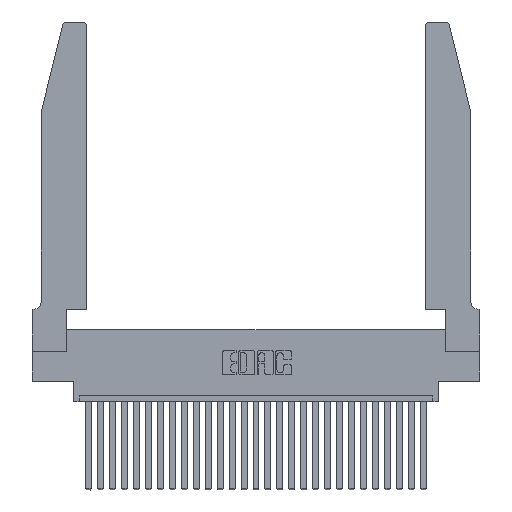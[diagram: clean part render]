
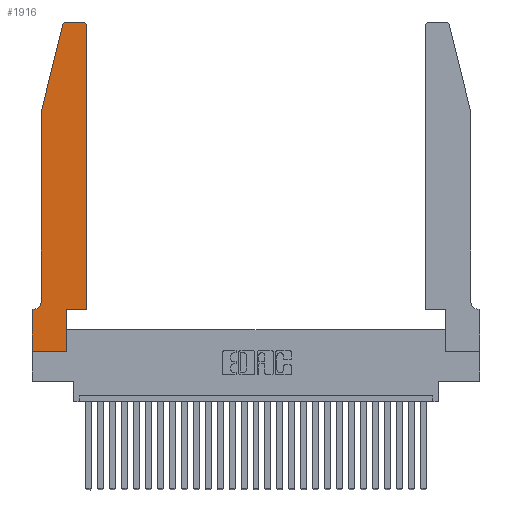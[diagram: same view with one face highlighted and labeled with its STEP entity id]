
A CAD part, top view. The second image highlights one B-rep face of the part: STEP entity #1916.
In plain terms, the highlighted planar face has unit normal (0, 0, 1).
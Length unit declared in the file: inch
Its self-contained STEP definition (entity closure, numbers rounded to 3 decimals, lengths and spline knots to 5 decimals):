
#500 = VERTEX_POINT ( 'NONE', #1086 ) ;
#628 = ORIENTED_EDGE ( 'NONE', *, *, #988, .T. ) ;
#988 = EDGE_CURVE ( 'NONE', #17002, #27458, #21247, .T. ) ;
#1086 = CARTESIAN_POINT ( 'NONE',  ( 0.0055, 0.35, 0.37 ) ) ;
#1126 = LINE ( 'NONE', #27932, #23735 ) ;
#1313 = DIRECTION ( 'NONE',  ( 0., 1., 0. ) ) ;
#1916 = ADVANCED_FACE ( 'NONE', ( #3417 ), #9056, .T. ) ;
#1995 = CARTESIAN_POINT ( 'NONE',  ( 0.4505, 0.35, 0.37 ) ) ;
#2101 = ORIENTED_EDGE ( 'NONE', *, *, #27405, .T. ) ;
#2316 = VECTOR ( 'NONE', #14322, 39.37008 ) ;
#2616 = CARTESIAN_POINT ( 'NONE',  ( 0.2605, 2.75, 0.37 ) ) ;
#2664 = DIRECTION ( 'NONE',  ( 0., -1., 0. ) ) ;
#3417 = FACE_OUTER_BOUND ( 'NONE', #25079, .T. ) ;
#3504 = EDGE_CURVE ( 'NONE', #11143, #8281, #8775, .T. ) ;
#3629 = DIRECTION ( 'NONE',  ( 0., 1., 0. ) ) ;
#4807 = EDGE_CURVE ( 'NONE', #21581, #500, #25152, .T. ) ;
#4892 = LINE ( 'NONE', #25205, #21672 ) ;
#4987 = DIRECTION ( 'NONE',  ( -1., 0., 0. ) ) ;
#4996 = CARTESIAN_POINT ( 'NONE',  ( 0.0755, 2., 0.37 ) ) ;
#5519 = AXIS2_PLACEMENT_3D ( 'NONE', #13324, #24188, #26760 ) ;
#5520 = VERTEX_POINT ( 'NONE', #14639 ) ;
#5659 = LINE ( 'NONE', #10145, #27556 ) ;
#5723 = ORIENTED_EDGE ( 'NONE', *, *, #15871, .T. ) ;
#5845 = CIRCLE ( 'NONE', #5519, 0.03 ) ;
#6104 = CARTESIAN_POINT ( 'NONE',  ( 0.4505, 0.35, 0.37 ) ) ;
#6282 = LINE ( 'NONE', #14754, #7245 ) ;
#7245 = VECTOR ( 'NONE', #10486, 39.37008 ) ;
#7622 = CARTESIAN_POINT ( 'NONE',  ( 0.2865, 0.35, 0.37 ) ) ;
#7676 = ORIENTED_EDGE ( 'NONE', *, *, #24217, .T. ) ;
#7936 = DIRECTION ( 'NONE',  ( -1., 0., 0. ) ) ;
#8152 = EDGE_CURVE ( 'NONE', #5520, #20333, #20514, .T. ) ;
#8167 = VERTEX_POINT ( 'NONE', #1995 ) ;
#8184 = DIRECTION ( 'NONE',  ( 1., 0., 0. ) ) ;
#8281 = VERTEX_POINT ( 'NONE', #17832 ) ;
#8543 = DIRECTION ( 'NONE',  ( 0., 0., 1. ) ) ;
#8602 = CARTESIAN_POINT ( 'NONE',  ( 0.0755, 0.42, 0.37 ) ) ;
#8775 = LINE ( 'NONE', #27477, #2316 ) ;
#9056 = PLANE ( 'NONE',  #27855 ) ;
#10145 = CARTESIAN_POINT ( 'NONE',  ( 0., 0., 0.37 ) ) ;
#10486 = DIRECTION ( 'NONE',  ( -0.239, -0.971, 0. ) ) ;
#10800 = CARTESIAN_POINT ( 'NONE',  ( 0., 0.35, 0.37 ) ) ;
#11143 = VERTEX_POINT ( 'NONE', #21629 ) ;
#11714 = LINE ( 'NONE', #6104, #22681 ) ;
#12067 = ORIENTED_EDGE ( 'NONE', *, *, #3504, .T. ) ;
#12732 = DIRECTION ( 'NONE',  ( 1., 0., 0. ) ) ;
#13299 = VECTOR ( 'NONE', #4987, 39.37008 ) ;
#13324 = CARTESIAN_POINT ( 'NONE',  ( 0.284, 2.72, 0.37 ) ) ;
#13483 = ORIENTED_EDGE ( 'NONE', *, *, #20026, .T. ) ;
#13984 = ORIENTED_EDGE ( 'NONE', *, *, #26946, .T. ) ;
#14322 = DIRECTION ( 'NONE',  ( 0., -1., 0. ) ) ;
#14639 = CARTESIAN_POINT ( 'NONE',  ( 0.2865, 0., 0.37 ) ) ;
#14754 = CARTESIAN_POINT ( 'NONE',  ( 0.0755, 2., 0.37 ) ) ;
#15560 = VERTEX_POINT ( 'NONE', #4996 ) ;
#15871 = EDGE_CURVE ( 'NONE', #27236, #17002, #22140, .T. ) ;
#16231 = ORIENTED_EDGE ( 'NONE', *, *, #4807, .T. ) ;
#17002 = VERTEX_POINT ( 'NONE', #25467 ) ;
#17112 = AXIS2_PLACEMENT_3D ( 'NONE', #27956, #8543, #12732 ) ;
#17244 = EDGE_CURVE ( 'NONE', #8281, #5520, #5659, .T. ) ;
#17595 = ORIENTED_EDGE ( 'NONE', *, *, #25597, .T. ) ;
#17832 = CARTESIAN_POINT ( 'NONE',  ( 0., 0., 0.37 ) ) ;
#18842 = CARTESIAN_POINT ( 'NONE',  ( 0.0055, 0.42, 0.37 ) ) ;
#19452 = VECTOR ( 'NONE', #2664, 39.37008 ) ;
#19632 = DIRECTION ( 'NONE',  ( 1., 0., 0. ) ) ;
#20026 = EDGE_CURVE ( 'NONE', #15560, #21581, #26980, .T. ) ;
#20333 = VERTEX_POINT ( 'NONE', #7622 ) ;
#20514 = LINE ( 'NONE', #21099, #23977 ) ;
#20959 = DIRECTION ( 'NONE',  ( 0., 0., -1. ) ) ;
#21099 = CARTESIAN_POINT ( 'NONE',  ( 0.2865, 0.35, 0.37 ) ) ;
#21247 = LINE ( 'NONE', #2616, #13299 ) ;
#21581 = VERTEX_POINT ( 'NONE', #8602 ) ;
#21629 = CARTESIAN_POINT ( 'NONE',  ( 0., 0.35, 0.37 ) ) ;
#21672 = VECTOR ( 'NONE', #3629, 39.37008 ) ;
#21818 = DIRECTION ( 'NONE',  ( 0., 0., 1. ) ) ;
#22140 = CIRCLE ( 'NONE', #17112, 0.03 ) ;
#22452 = CARTESIAN_POINT ( 'NONE',  ( 0.4505, 2.72, 0.37 ) ) ;
#22681 = VECTOR ( 'NONE', #8184, 39.37008 ) ;
#23303 = DIRECTION ( 'NONE',  ( -1., 0., 0. ) ) ;
#23526 = CARTESIAN_POINT ( 'NONE',  ( 0.284, 2.75, 0.37 ) ) ;
#23735 = VECTOR ( 'NONE', #23303, 39.37008 ) ;
#23977 = VECTOR ( 'NONE', #1313, 39.37008 ) ;
#24188 = DIRECTION ( 'NONE',  ( 0., 0., 1. ) ) ;
#24217 = EDGE_CURVE ( 'NONE', #20333, #8167, #11714, .T. ) ;
#25079 = EDGE_LOOP ( 'NONE', ( #628, #17595, #13984, #13483, #16231, #27061, #12067, #25663, #28019, #7676, #2101, #5723 ) ) ;
#25152 = CIRCLE ( 'NONE', #26424, 0.07 ) ;
#25205 = CARTESIAN_POINT ( 'NONE',  ( 0.4505, 0.35, 0.37 ) ) ;
#25322 = VERTEX_POINT ( 'NONE', #27359 ) ;
#25467 = CARTESIAN_POINT ( 'NONE',  ( 0.4205, 2.75, 0.37 ) ) ;
#25597 = EDGE_CURVE ( 'NONE', #27458, #25322, #5845, .T. ) ;
#25663 = ORIENTED_EDGE ( 'NONE', *, *, #17244, .T. ) ;
#26124 = DIRECTION ( 'NONE',  ( 1., 0., 0. ) ) ;
#26203 = EDGE_CURVE ( 'NONE', #500, #11143, #1126, .T. ) ;
#26424 = AXIS2_PLACEMENT_3D ( 'NONE', #18842, #20959, #7936 ) ;
#26732 = CARTESIAN_POINT ( 'NONE',  ( 0.0755, 2., 0.37 ) ) ;
#26760 = DIRECTION ( 'NONE',  ( 1., 0., 0. ) ) ;
#26946 = EDGE_CURVE ( 'NONE', #25322, #15560, #6282, .T. ) ;
#26980 = LINE ( 'NONE', #26732, #19452 ) ;
#27061 = ORIENTED_EDGE ( 'NONE', *, *, #26203, .T. ) ;
#27236 = VERTEX_POINT ( 'NONE', #22452 ) ;
#27359 = CARTESIAN_POINT ( 'NONE',  ( 0.25487, 2.72718, 0.37 ) ) ;
#27405 = EDGE_CURVE ( 'NONE', #8167, #27236, #4892, .T. ) ;
#27458 = VERTEX_POINT ( 'NONE', #23526 ) ;
#27477 = CARTESIAN_POINT ( 'NONE',  ( 0., 0., 0.37 ) ) ;
#27556 = VECTOR ( 'NONE', #19632, 39.37008 ) ;
#27855 = AXIS2_PLACEMENT_3D ( 'NONE', #10800, #21818, #26124 ) ;
#27932 = CARTESIAN_POINT ( 'NONE',  ( 0.0755, 0.35, 0.37 ) ) ;
#27956 = CARTESIAN_POINT ( 'NONE',  ( 0.4205, 2.72, 0.37 ) ) ;
#28019 = ORIENTED_EDGE ( 'NONE', *, *, #8152, .T. ) ;
